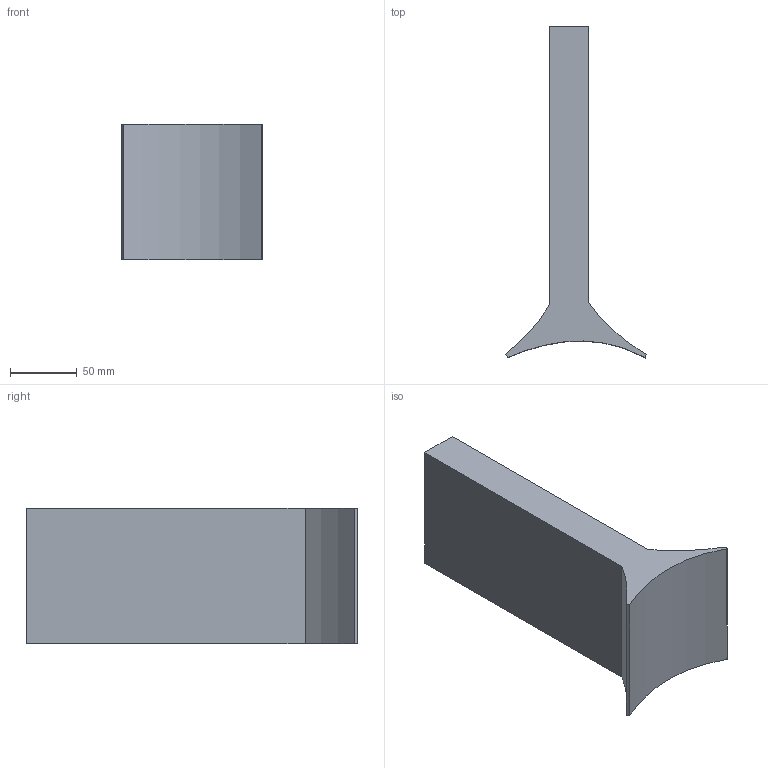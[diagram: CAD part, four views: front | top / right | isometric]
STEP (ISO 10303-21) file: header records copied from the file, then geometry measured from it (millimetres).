
FILE_DESCRIPTION (( 'STEP AP214' ), '1' );
FILE_NAME ('Pusher.STEP', '2014-02-05T15:25:14', ( 'elpi' ), ( '' ), 'SwSTEP 2.0', 'SolidWorks 2013', '' );
FILE_SCHEMA (( 'AUTOMOTIVE_DESIGN' ));
Length unit declared in the file: inch
Products named in the file (1): Pusher
Bounding box: 105.39 x 248.7 x 101.6 mm (x, y, z)
Volume: 799723.9 mm3; surface area: 83508.2 mm2
Topology: 1 solids, 1 shells, 11 faces, 27 edges, 18 vertices
Faces by surface type: plane 5, cylinder 3, bspline 3
Entity records: 373 total; most frequent: CARTESIAN_POINT 84, ORIENTED_EDGE 54, DIRECTION 45, EDGE_CURVE 27, VERTEX_POINT 18, LINE 15, VECTOR 15, AXIS2_PLACEMENT_3D 15
